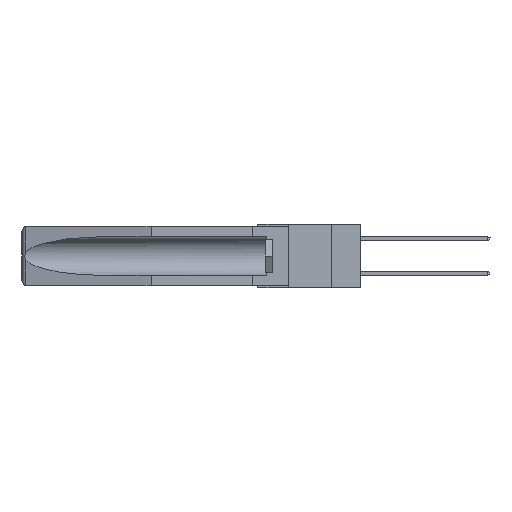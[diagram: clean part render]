
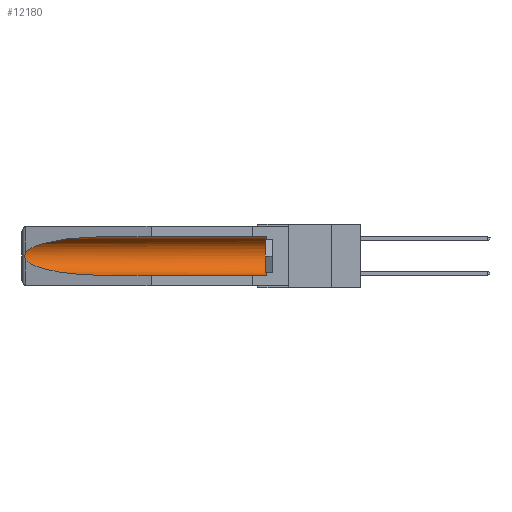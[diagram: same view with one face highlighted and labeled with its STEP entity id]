
A CAD part, left-side view. The second image highlights one B-rep face of the part: STEP entity #12180.
In plain terms, the highlighted cylindrical face has radius 2.857 mm (diameter 5.715 mm), a partial arc.
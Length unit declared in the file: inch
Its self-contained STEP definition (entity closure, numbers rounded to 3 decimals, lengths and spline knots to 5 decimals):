
#3 = CARTESIAN_POINT ( 'NONE',  ( 0.2673, 1.5327, -0.16383 ) ) ;
#91 =( BOUNDED_CURVE ( )  B_SPLINE_CURVE ( 3, ( #9824, #216, #8187, #14921 ),
 .UNSPECIFIED., .F., .F. ) 
 B_SPLINE_CURVE_WITH_KNOTS ( ( 4, 4 ),
 ( 4.71239, 6.08839 ),
 .UNSPECIFIED. ) 
 CURVE ( )  GEOMETRIC_REPRESENTATION_ITEM ( )  RATIONAL_B_SPLINE_CURVE ( ( 1., 0.848, 0.848, 1. ) ) 
 REPRESENTATION_ITEM ( '' )  );
#216 = CARTESIAN_POINT ( 'NONE',  ( 0.21114, 1.30732, -0.059 ) ) ;
#224 = VERTEX_POINT ( 'NONE', #13440 ) ;
#777 = DIRECTION ( 'NONE',  ( 0., -1., 0. ) ) ;
#850 = CIRCLE ( 'NONE', #13738, 0.1125 ) ;
#1914 = CARTESIAN_POINT ( 'NONE',  ( 0.26537, 1.52718, -0.19328 ) ) ;
#1938 =( BOUNDED_CURVE ( )  B_SPLINE_CURVE ( 3, ( #19485, #11390, #3292, #13090 ),
 .UNSPECIFIED., .F., .T. ) 
 B_SPLINE_CURVE_WITH_KNOTS ( ( 4, 4 ),
 ( 0.1948, 1.5708 ),
 .UNSPECIFIED. ) 
 CURVE ( )  GEOMETRIC_REPRESENTATION_ITEM ( )  RATIONAL_B_SPLINE_CURVE ( ( 1., 0.848, 0.848, 1. ) ) 
 REPRESENTATION_ITEM ( '' )  );
#2040 = EDGE_CURVE ( 'NONE', #7783, #10408, #11001, .T. ) ;
#2467 = EDGE_CURVE ( 'NONE', #7783, #15775, #850, .T. ) ;
#2474 = VERTEX_POINT ( 'NONE', #2618 ) ;
#2618 = CARTESIAN_POINT ( 'NONE',  ( 0.26537, 1.52718, -0.19328 ) ) ;
#3011 = DIRECTION ( 'NONE',  ( 0., 1., 0. ) ) ;
#3146 = LINE ( 'NONE', #10917, #6658 ) ;
#3204 = EDGE_CURVE ( 'NONE', #15775, #224, #3146, .T. ) ;
#3292 = CARTESIAN_POINT ( 'NONE',  ( 0.21114, 1.30732, -0.284 ) ) ;
#3423 = CARTESIAN_POINT ( 'NONE',  ( 0.155, 0.126, -0.059 ) ) ;
#3507 = ORIENTED_EDGE ( 'NONE', *, *, #13879, .T. ) ;
#5335 = CARTESIAN_POINT ( 'NONE',  ( 0.155, 0.126, -0.284 ) ) ;
#6494 = CARTESIAN_POINT ( 'NONE',  ( 0.26654, 1.53092, -0.15636 ) ) ;
#6658 = VECTOR ( 'NONE', #3011, 39.37008 ) ;
#6696 = VECTOR ( 'NONE', #15915, 39.37008 ) ;
#7783 = VERTEX_POINT ( 'NONE', #5335 ) ;
#8121 = CARTESIAN_POINT ( 'NONE',  ( 0.2675, 1.53308, -0.17534 ) ) ;
#8157 = ORIENTED_EDGE ( 'NONE', *, *, #11170, .T. ) ;
#8187 = CARTESIAN_POINT ( 'NONE',  ( 0.25451, 1.48313, -0.09465 ) ) ;
#9736 = CARTESIAN_POINT ( 'NONE',  ( 0.26655, 1.53094, -0.18657 ) ) ;
#9824 = CARTESIAN_POINT ( 'NONE',  ( 0.155, 1.07973, -0.059 ) ) ;
#10408 = VERTEX_POINT ( 'NONE', #14458 ) ;
#10742 = CARTESIAN_POINT ( 'NONE',  ( 0.155, -0.30754, -0.1715 ) ) ;
#10917 = CARTESIAN_POINT ( 'NONE',  ( 0.155, -0.30754, -0.059 ) ) ;
#11001 = LINE ( 'NONE', #14493, #6696 ) ;
#11170 = EDGE_CURVE ( 'NONE', #12477, #2474, #17882, .T. ) ;
#11362 = CARTESIAN_POINT ( 'NONE',  ( 0.26597, 1.5296, -0.19026 ) ) ;
#11390 = CARTESIAN_POINT ( 'NONE',  ( 0.25451, 1.48313, -0.24835 ) ) ;
#11786 = ORIENTED_EDGE ( 'NONE', *, *, #3204, .T. ) ;
#11932 = ORIENTED_EDGE ( 'NONE', *, *, #2040, .F. ) ;
#12066 = DIRECTION ( 'NONE',  ( 0., 0., 1. ) ) ;
#12180 = ADVANCED_FACE ( 'NONE', ( #19084 ), #15267, .F. ) ;
#12377 = ORIENTED_EDGE ( 'NONE', *, *, #2467, .T. ) ;
#12433 = DIRECTION ( 'NONE',  ( 0., 1., 0. ) ) ;
#12457 = EDGE_LOOP ( 'NONE', ( #13549, #8157, #3507, #11932, #12377, #11786 ) ) ;
#12477 = VERTEX_POINT ( 'NONE', #13941 ) ;
#13090 = CARTESIAN_POINT ( 'NONE',  ( 0.155, 1.07973, -0.284 ) ) ;
#13440 = CARTESIAN_POINT ( 'NONE',  ( 0.155, 1.07973, -0.059 ) ) ;
#13549 = ORIENTED_EDGE ( 'NONE', *, *, #14373, .T. ) ;
#13738 = AXIS2_PLACEMENT_3D ( 'NONE', #20227, #777, #12066 ) ;
#13879 = EDGE_CURVE ( 'NONE', #2474, #10408, #1938, .T. ) ;
#13941 = CARTESIAN_POINT ( 'NONE',  ( 0.26537, 1.52718, -0.14972 ) ) ;
#14111 = AXIS2_PLACEMENT_3D ( 'NONE', #10742, #12433, #18876 ) ;
#14373 = EDGE_CURVE ( 'NONE', #224, #12477, #91, .T. ) ;
#14458 = CARTESIAN_POINT ( 'NONE',  ( 0.155, 1.07973, -0.284 ) ) ;
#14493 = CARTESIAN_POINT ( 'NONE',  ( 0.155, -0.30754, -0.284 ) ) ;
#14921 = CARTESIAN_POINT ( 'NONE',  ( 0.26537, 1.52718, -0.14972 ) ) ;
#15267 = CYLINDRICAL_SURFACE ( 'NONE', #14111, 0.1125 ) ;
#15775 = VERTEX_POINT ( 'NONE', #3423 ) ;
#15915 = DIRECTION ( 'NONE',  ( 0., 1., 0. ) ) ;
#17822 = CARTESIAN_POINT ( 'NONE',  ( 0.2675, 1.53308, -0.16763 ) ) ;
#17882 = B_SPLINE_CURVE_WITH_KNOTS ( 'NONE', 3,
 ( #18032, #19523, #6494, #3, #17822, #8121, #19458, #9736, #11362, #1914 ),
 .UNSPECIFIED., .F., .F.,
 ( 4, 2, 2, 2, 4 ),
 ( 0., 0.00029, 0.00058, 0.00087, 0.00117 ),
 .UNSPECIFIED. ) ;
#18032 = CARTESIAN_POINT ( 'NONE',  ( 0.26537, 1.52718, -0.14972 ) ) ;
#18876 = DIRECTION ( 'NONE',  ( 0., 0., 1. ) ) ;
#19084 = FACE_OUTER_BOUND ( 'NONE', #12457, .T. ) ;
#19458 = CARTESIAN_POINT ( 'NONE',  ( 0.2673, 1.53269, -0.17917 ) ) ;
#19485 = CARTESIAN_POINT ( 'NONE',  ( 0.26537, 1.52718, -0.19328 ) ) ;
#19523 = CARTESIAN_POINT ( 'NONE',  ( 0.26597, 1.52961, -0.15275 ) ) ;
#20227 = CARTESIAN_POINT ( 'NONE',  ( 0.155, 0.126, -0.1715 ) ) ;
